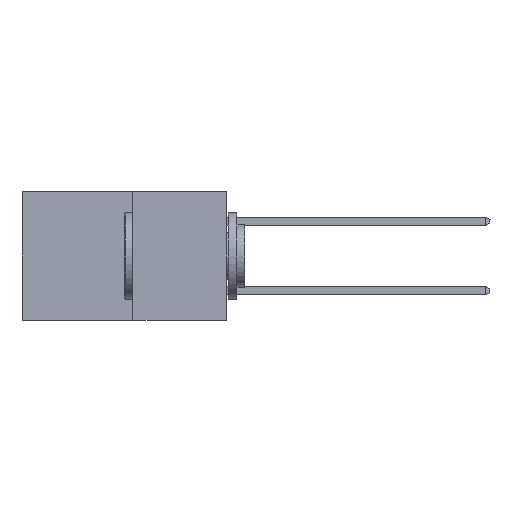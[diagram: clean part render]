
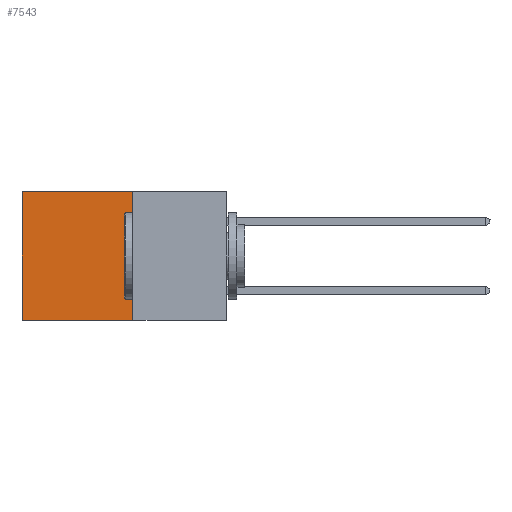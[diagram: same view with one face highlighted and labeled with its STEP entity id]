
A CAD part, left-side view. The second image highlights one B-rep face of the part: STEP entity #7543.
In plain terms, the highlighted planar face has unit normal (-1, 0, 0).
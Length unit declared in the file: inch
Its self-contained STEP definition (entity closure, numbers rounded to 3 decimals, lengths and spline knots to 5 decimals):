
#651 = PLANE ( 'NONE',  #1056 ) ;
#966 = ORIENTED_EDGE ( 'NONE', *, *, #11236, .F. ) ;
#1056 = AXIS2_PLACEMENT_3D ( 'NONE', #10567, #11679, #5095 ) ;
#1654 = CARTESIAN_POINT ( 'NONE',  ( 0.277, 0.59, -0.37 ) ) ;
#2555 = VECTOR ( 'NONE', #13940, 39.37008 ) ;
#2607 = VERTEX_POINT ( 'NONE', #12962 ) ;
#2728 = VERTEX_POINT ( 'NONE', #12116 ) ;
#3821 = CARTESIAN_POINT ( 'NONE',  ( 0.277, 0.27, -0.37 ) ) ;
#4096 = CARTESIAN_POINT ( 'NONE',  ( 0.277, 0.27, -0.37 ) ) ;
#4107 = LINE ( 'NONE', #8021, #12538 ) ;
#4501 = VERTEX_POINT ( 'NONE', #10178 ) ;
#4608 = EDGE_CURVE ( 'NONE', #2728, #12662, #4107, .T. ) ;
#5095 = DIRECTION ( 'NONE',  ( 0., 0., -1. ) ) ;
#5247 = VECTOR ( 'NONE', #10688, 39.37008 ) ;
#5281 = ORIENTED_EDGE ( 'NONE', *, *, #6958, .F. ) ;
#5372 = EDGE_CURVE ( 'NONE', #2607, #2728, #5466, .T. ) ;
#5378 = VECTOR ( 'NONE', #13699, 39.37008 ) ;
#5466 = LINE ( 'NONE', #7566, #2555 ) ;
#6958 = EDGE_CURVE ( 'NONE', #2607, #4501, #13657, .T. ) ;
#7543 = ADVANCED_FACE ( 'NONE', ( #11938 ), #651, .F. ) ;
#7566 = CARTESIAN_POINT ( 'NONE',  ( 0.277, 0.27, 0. ) ) ;
#8021 = CARTESIAN_POINT ( 'NONE',  ( 0.277, 0.59, -0.37 ) ) ;
#8362 = ORIENTED_EDGE ( 'NONE', *, *, #4608, .T. ) ;
#9631 = DIRECTION ( 'NONE',  ( 0., 0., -1. ) ) ;
#10178 = CARTESIAN_POINT ( 'NONE',  ( 0.277, 0.27, -0.37 ) ) ;
#10567 = CARTESIAN_POINT ( 'NONE',  ( 0.277, 0.27, -0.37 ) ) ;
#10688 = DIRECTION ( 'NONE',  ( 0., 0., -1. ) ) ;
#11006 = EDGE_LOOP ( 'NONE', ( #8362, #966, #5281, #12507 ) ) ;
#11236 = EDGE_CURVE ( 'NONE', #4501, #12662, #14119, .T. ) ;
#11679 = DIRECTION ( 'NONE',  ( 1., 0., 0. ) ) ;
#11938 = FACE_OUTER_BOUND ( 'NONE', #11006, .T. ) ;
#12116 = CARTESIAN_POINT ( 'NONE',  ( 0.277, 0.59, 0. ) ) ;
#12507 = ORIENTED_EDGE ( 'NONE', *, *, #5372, .T. ) ;
#12538 = VECTOR ( 'NONE', #9631, 39.37008 ) ;
#12662 = VERTEX_POINT ( 'NONE', #1654 ) ;
#12962 = CARTESIAN_POINT ( 'NONE',  ( 0.277, 0.27, 0. ) ) ;
#13657 = LINE ( 'NONE', #4096, #5247 ) ;
#13699 = DIRECTION ( 'NONE',  ( 0., 1., 0. ) ) ;
#13940 = DIRECTION ( 'NONE',  ( 0., 1., 0. ) ) ;
#14119 = LINE ( 'NONE', #3821, #5378 ) ;
